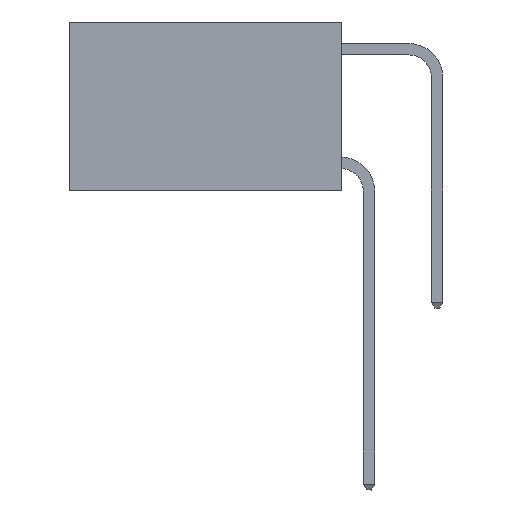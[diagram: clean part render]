
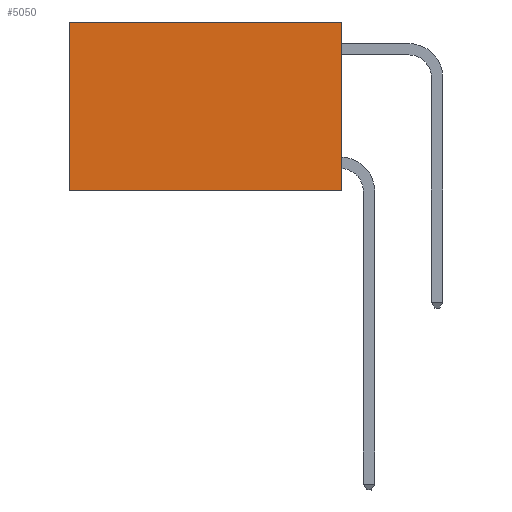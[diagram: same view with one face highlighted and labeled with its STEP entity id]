
A CAD part, left-side view. The second image highlights one B-rep face of the part: STEP entity #5050.
In plain terms, the highlighted planar face has unit normal (-1, 0, 0).
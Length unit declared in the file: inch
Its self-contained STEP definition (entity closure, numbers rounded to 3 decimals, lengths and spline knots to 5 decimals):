
#94 = VERTEX_POINT ( 'NONE', #1999 ) ;
#363 = CARTESIAN_POINT ( 'NONE',  ( 0.2625, 0., -0.37 ) ) ;
#532 = CARTESIAN_POINT ( 'NONE',  ( 0.2625, 0., 0. ) ) ;
#841 = EDGE_CURVE ( 'NONE', #9759, #94, #9856, .T. ) ;
#928 = VERTEX_POINT ( 'NONE', #6762 ) ;
#1200 = ORIENTED_EDGE ( 'NONE', *, *, #9977, .F. ) ;
#1337 = DIRECTION ( 'NONE',  ( 0., 0., -1. ) ) ;
#1371 = DIRECTION ( 'NONE',  ( 0., 0., -1. ) ) ;
#1628 = FACE_OUTER_BOUND ( 'NONE', #1967, .T. ) ;
#1967 = EDGE_LOOP ( 'NONE', ( #6691, #6496, #1200, #1972 ) ) ;
#1972 = ORIENTED_EDGE ( 'NONE', *, *, #841, .T. ) ;
#1999 = CARTESIAN_POINT ( 'NONE',  ( 0.2625, 0.6, 0. ) ) ;
#2003 = DIRECTION ( 'NONE',  ( 0., 1., 0. ) ) ;
#2477 = LINE ( 'NONE', #363, #8589 ) ;
#2930 = CARTESIAN_POINT ( 'NONE',  ( 0.2625, 0., 0. ) ) ;
#3289 = LINE ( 'NONE', #2930, #9331 ) ;
#3726 = PLANE ( 'NONE',  #8149 ) ;
#4472 = DIRECTION ( 'NONE',  ( 0., 0., -1. ) ) ;
#5050 = ADVANCED_FACE ( 'NONE', ( #1628 ), #3726, .F. ) ;
#5379 = CARTESIAN_POINT ( 'NONE',  ( 0.2625, 0., 0. ) ) ;
#6000 = CARTESIAN_POINT ( 'NONE',  ( 0.2625, 0., 0. ) ) ;
#6043 = EDGE_CURVE ( 'NONE', #928, #7245, #2477, .T. ) ;
#6067 = VECTOR ( 'NONE', #9519, 39.37008 ) ;
#6234 = DIRECTION ( 'NONE',  ( 1., 0., 0. ) ) ;
#6496 = ORIENTED_EDGE ( 'NONE', *, *, #6043, .F. ) ;
#6691 = ORIENTED_EDGE ( 'NONE', *, *, #8236, .T. ) ;
#6762 = CARTESIAN_POINT ( 'NONE',  ( 0.2625, 0., -0.37 ) ) ;
#6772 = VECTOR ( 'NONE', #4472, 39.37008 ) ;
#6910 = CARTESIAN_POINT ( 'NONE',  ( 0.2625, 0.6, 0. ) ) ;
#7245 = VERTEX_POINT ( 'NONE', #8065 ) ;
#7850 = LINE ( 'NONE', #6910, #6772 ) ;
#8065 = CARTESIAN_POINT ( 'NONE',  ( 0.2625, 0.6, -0.37 ) ) ;
#8149 = AXIS2_PLACEMENT_3D ( 'NONE', #532, #6234, #1371 ) ;
#8236 = EDGE_CURVE ( 'NONE', #94, #7245, #7850, .T. ) ;
#8589 = VECTOR ( 'NONE', #2003, 39.37008 ) ;
#9331 = VECTOR ( 'NONE', #1337, 39.37008 ) ;
#9519 = DIRECTION ( 'NONE',  ( 0., 1., 0. ) ) ;
#9759 = VERTEX_POINT ( 'NONE', #6000 ) ;
#9856 = LINE ( 'NONE', #5379, #6067 ) ;
#9977 = EDGE_CURVE ( 'NONE', #9759, #928, #3289, .T. ) ;
